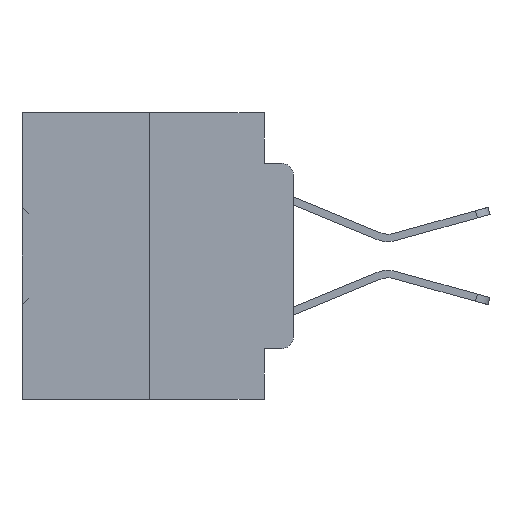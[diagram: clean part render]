
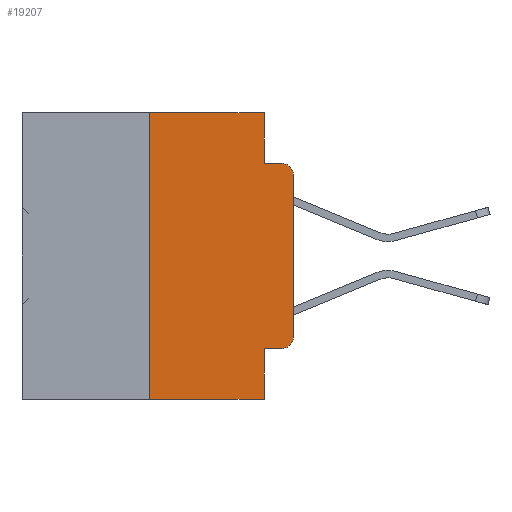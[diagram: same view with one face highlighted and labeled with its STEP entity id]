
A CAD part, left-side view. The second image highlights one B-rep face of the part: STEP entity #19207.
In plain terms, the highlighted planar face has unit normal (-1, 0, 0).
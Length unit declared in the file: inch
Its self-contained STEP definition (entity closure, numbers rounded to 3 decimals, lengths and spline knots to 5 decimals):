
#394 = ORIENTED_EDGE ( 'NONE', *, *, #23838, .T. ) ;
#781 = VERTEX_POINT ( 'NONE', #8207 ) ;
#926 = LINE ( 'NONE', #28075, #8267 ) ;
#1133 = VERTEX_POINT ( 'NONE', #11263 ) ;
#2317 = CARTESIAN_POINT ( 'NONE',  ( 0., 0.25, 0. ) ) ;
#2411 = EDGE_CURVE ( 'NONE', #19077, #781, #33064, .T. ) ;
#2947 = CARTESIAN_POINT ( 'NONE',  ( 0., 0.473, -0.5 ) ) ;
#3659 = VERTEX_POINT ( 'NONE', #2317 ) ;
#4281 = ORIENTED_EDGE ( 'NONE', *, *, #10803, .T. ) ;
#4554 = EDGE_CURVE ( 'NONE', #781, #27015, #23229, .T. ) ;
#4817 = LINE ( 'NONE', #8939, #20374 ) ;
#5775 = ORIENTED_EDGE ( 'NONE', *, *, #21977, .F. ) ;
#6102 = DIRECTION ( 'NONE',  ( 0., -1., 0. ) ) ;
#6683 = VECTOR ( 'NONE', #19305, 39.37008 ) ;
#7098 = VERTEX_POINT ( 'NONE', #11594 ) ;
#7313 = ORIENTED_EDGE ( 'NONE', *, *, #28237, .T. ) ;
#8207 = CARTESIAN_POINT ( 'NONE',  ( 0., 0.051, -0.0885 ) ) ;
#8267 = VECTOR ( 'NONE', #31186, 39.37008 ) ;
#8291 = ORIENTED_EDGE ( 'NONE', *, *, #8690, .T. ) ;
#8296 = VECTOR ( 'NONE', #18207, 39.37008 ) ;
#8418 = LINE ( 'NONE', #35702, #9396 ) ;
#8468 = CARTESIAN_POINT ( 'NONE',  ( 0., 0., -0.3915 ) ) ;
#8690 = EDGE_CURVE ( 'NONE', #19215, #27015, #12931, .T. ) ;
#8939 = CARTESIAN_POINT ( 'NONE',  ( 0., 0.051, -0.4115 ) ) ;
#9396 = VECTOR ( 'NONE', #17189, 39.37008 ) ;
#10803 = EDGE_CURVE ( 'NONE', #36666, #19215, #12820, .T. ) ;
#11214 = DIRECTION ( 'NONE',  ( -1., 0., 0. ) ) ;
#11263 = CARTESIAN_POINT ( 'NONE',  ( 0., 0.02, -0.4115 ) ) ;
#11594 = CARTESIAN_POINT ( 'NONE',  ( 0., 0.051, -0.5 ) ) ;
#11711 = CARTESIAN_POINT ( 'NONE',  ( 0., 0.051, 0. ) ) ;
#11804 = VECTOR ( 'NONE', #18534, 39.37008 ) ;
#12392 = DIRECTION ( 'NONE',  ( 0., 0., -1. ) ) ;
#12820 = LINE ( 'NONE', #33957, #11804 ) ;
#12931 = CIRCLE ( 'NONE', #16125, 0.02 ) ;
#14199 = LINE ( 'NONE', #2947, #29740 ) ;
#15428 = CARTESIAN_POINT ( 'NONE',  ( 0., 0.051, -0.4115 ) ) ;
#16125 = AXIS2_PLACEMENT_3D ( 'NONE', #29819, #11214, #32917 ) ;
#16892 = EDGE_LOOP ( 'NONE', ( #4281, #8291, #32013, #30580, #5775, #17586, #394, #34867, #24326, #7313 ) ) ;
#17189 = DIRECTION ( 'NONE',  ( 0., -1., 0. ) ) ;
#17586 = ORIENTED_EDGE ( 'NONE', *, *, #38480, .F. ) ;
#18141 = DIRECTION ( 'NONE',  ( -1., 0., 0. ) ) ;
#18207 = DIRECTION ( 'NONE',  ( 0., 0., -1. ) ) ;
#18534 = DIRECTION ( 'NONE',  ( 0., 0., 1. ) ) ;
#18539 = VERTEX_POINT ( 'NONE', #15428 ) ;
#19077 = VERTEX_POINT ( 'NONE', #11711 ) ;
#19207 = ADVANCED_FACE ( 'NONE', ( #24641 ), #27861, .F. ) ;
#19215 = VERTEX_POINT ( 'NONE', #37109 ) ;
#19305 = DIRECTION ( 'NONE',  ( 0., -1., 0. ) ) ;
#20374 = VECTOR ( 'NONE', #21343, 39.37008 ) ;
#21046 = AXIS2_PLACEMENT_3D ( 'NONE', #40047, #30985, #12392 ) ;
#21225 = CARTESIAN_POINT ( 'NONE',  ( 0., 0.02, -0.0885 ) ) ;
#21343 = DIRECTION ( 'NONE',  ( 0., -1., 0. ) ) ;
#21677 = CARTESIAN_POINT ( 'NONE',  ( 0., 0.25, 0. ) ) ;
#21977 = EDGE_CURVE ( 'NONE', #3659, #19077, #8418, .T. ) ;
#22670 = VERTEX_POINT ( 'NONE', #38713 ) ;
#23229 = LINE ( 'NONE', #31779, #6683 ) ;
#23838 = EDGE_CURVE ( 'NONE', #22670, #7098, #14199, .T. ) ;
#24326 = ORIENTED_EDGE ( 'NONE', *, *, #30313, .T. ) ;
#24487 = CARTESIAN_POINT ( 'NONE',  ( 0., 0.051, 0. ) ) ;
#24641 = FACE_OUTER_BOUND ( 'NONE', #16892, .T. ) ;
#24815 = DIRECTION ( 'NONE',  ( 0., 0., 1. ) ) ;
#27015 = VERTEX_POINT ( 'NONE', #21225 ) ;
#27861 = PLANE ( 'NONE',  #21046 ) ;
#28075 = CARTESIAN_POINT ( 'NONE',  ( 0., 0.051, 0. ) ) ;
#28237 = EDGE_CURVE ( 'NONE', #1133, #36666, #37427, .T. ) ;
#29589 = VECTOR ( 'NONE', #24815, 39.37008 ) ;
#29740 = VECTOR ( 'NONE', #6102, 39.37008 ) ;
#29819 = CARTESIAN_POINT ( 'NONE',  ( 0., 0.02, -0.1085 ) ) ;
#30313 = EDGE_CURVE ( 'NONE', #18539, #1133, #4817, .T. ) ;
#30580 = ORIENTED_EDGE ( 'NONE', *, *, #2411, .F. ) ;
#30985 = DIRECTION ( 'NONE',  ( 1., 0., 0. ) ) ;
#31186 = DIRECTION ( 'NONE',  ( 0., 0., -1. ) ) ;
#31264 = AXIS2_PLACEMENT_3D ( 'NONE', #36632, #18141, #39712 ) ;
#31779 = CARTESIAN_POINT ( 'NONE',  ( 0., 0.051, -0.0885 ) ) ;
#32013 = ORIENTED_EDGE ( 'NONE', *, *, #4554, .F. ) ;
#32917 = DIRECTION ( 'NONE',  ( 0., 0., -1. ) ) ;
#33064 = LINE ( 'NONE', #24487, #8296 ) ;
#33957 = CARTESIAN_POINT ( 'NONE',  ( 0., 0., 0. ) ) ;
#34405 = EDGE_CURVE ( 'NONE', #18539, #7098, #926, .T. ) ;
#34867 = ORIENTED_EDGE ( 'NONE', *, *, #34405, .F. ) ;
#35702 = CARTESIAN_POINT ( 'NONE',  ( 0., 0.473, 0. ) ) ;
#36632 = CARTESIAN_POINT ( 'NONE',  ( 0., 0.02, -0.3915 ) ) ;
#36666 = VERTEX_POINT ( 'NONE', #8468 ) ;
#37109 = CARTESIAN_POINT ( 'NONE',  ( 0., 0., -0.1085 ) ) ;
#37427 = CIRCLE ( 'NONE', #31264, 0.02 ) ;
#37711 = LINE ( 'NONE', #21677, #29589 ) ;
#38480 = EDGE_CURVE ( 'NONE', #22670, #3659, #37711, .T. ) ;
#38713 = CARTESIAN_POINT ( 'NONE',  ( 0., 0.25, -0.5 ) ) ;
#39712 = DIRECTION ( 'NONE',  ( 0., 0., -1. ) ) ;
#40047 = CARTESIAN_POINT ( 'NONE',  ( 0., 0.473, 0. ) ) ;
